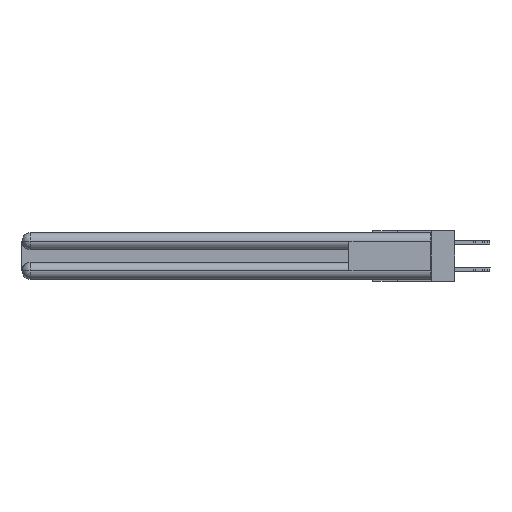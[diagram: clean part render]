
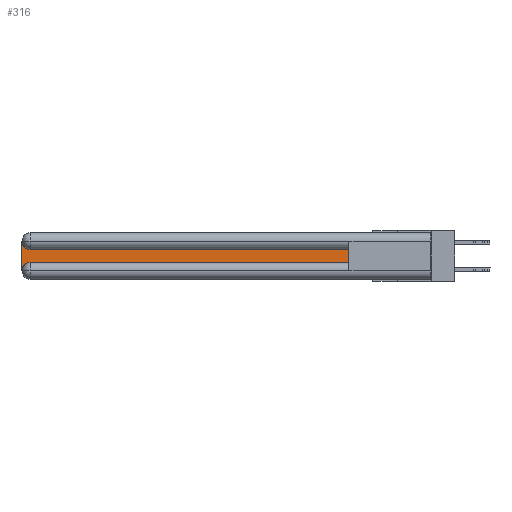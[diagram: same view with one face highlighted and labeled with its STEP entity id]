
A CAD part, left-side view. The second image highlights one B-rep face of the part: STEP entity #316.
In plain terms, the highlighted planar face has unit normal (-1, 0, 0).
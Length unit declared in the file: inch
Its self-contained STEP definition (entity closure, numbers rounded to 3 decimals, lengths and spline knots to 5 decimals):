
#155 = VERTEX_POINT ( 'NONE', #11225 ) ;
#316 = ADVANCED_FACE ( 'NONE', ( #6992 ), #21529, .F. ) ;
#781 = AXIS2_PLACEMENT_3D ( 'NONE', #875, #32327, #5936 ) ;
#875 = CARTESIAN_POINT ( 'NONE',  ( 0.075, 3., -0.1225 ) ) ;
#1065 = LINE ( 'NONE', #25532, #20812 ) ;
#3081 = CARTESIAN_POINT ( 'NONE',  ( 0.075, 3., -0.2775 ) ) ;
#3190 = CARTESIAN_POINT ( 'NONE',  ( 0.075, 2.94, -0.1225 ) ) ;
#3646 = CIRCLE ( 'NONE', #11608, 0.06 ) ;
#3935 = CARTESIAN_POINT ( 'NONE',  ( 0.075, 0.6, -0.1225 ) ) ;
#4728 = DIRECTION ( 'NONE',  ( 0., -1., 0. ) ) ;
#5057 = VERTEX_POINT ( 'NONE', #25517 ) ;
#5254 = ORIENTED_EDGE ( 'NONE', *, *, #30267, .T. ) ;
#5693 = EDGE_CURVE ( 'NONE', #22349, #15448, #27275, .T. ) ;
#5936 = DIRECTION ( 'NONE',  ( 0., 0., -1. ) ) ;
#6857 = ORIENTED_EDGE ( 'NONE', *, *, #26820, .T. ) ;
#6992 = FACE_OUTER_BOUND ( 'NONE', #21489, .T. ) ;
#7317 = CARTESIAN_POINT ( 'NONE',  ( 0.075, 3., -0.0625 ) ) ;
#7376 = CARTESIAN_POINT ( 'NONE',  ( 0.075, 2.94, -0.2775 ) ) ;
#8528 = EDGE_CURVE ( 'NONE', #155, #13102, #28706, .T. ) ;
#10311 = DIRECTION ( 'NONE',  ( 0., 0., -1. ) ) ;
#10368 = DIRECTION ( 'NONE',  ( 1., 0., 0. ) ) ;
#11192 = LINE ( 'NONE', #20145, #24390 ) ;
#11225 = CARTESIAN_POINT ( 'NONE',  ( 0.075, 0.6, -0.2175 ) ) ;
#11458 = ORIENTED_EDGE ( 'NONE', *, *, #5693, .T. ) ;
#11608 = AXIS2_PLACEMENT_3D ( 'NONE', #7376, #30932, #10311 ) ;
#11888 = LINE ( 'NONE', #3935, #13582 ) ;
#13102 = VERTEX_POINT ( 'NONE', #32010 ) ;
#13129 = VERTEX_POINT ( 'NONE', #3081 ) ;
#13582 = VECTOR ( 'NONE', #15214, 39.37008 ) ;
#13713 = AXIS2_PLACEMENT_3D ( 'NONE', #15583, #10368, #28789 ) ;
#15214 = DIRECTION ( 'NONE',  ( 0., 1., 0. ) ) ;
#15448 = VERTEX_POINT ( 'NONE', #7317 ) ;
#15583 = CARTESIAN_POINT ( 'NONE',  ( 0.075, 2.94, -0.0625 ) ) ;
#20145 = CARTESIAN_POINT ( 'NONE',  ( 0.075, 0.6, -0.2175 ) ) ;
#20575 = EDGE_CURVE ( 'NONE', #15448, #13129, #1065, .T. ) ;
#20812 = VECTOR ( 'NONE', #28038, 39.37008 ) ;
#21489 = EDGE_LOOP ( 'NONE', ( #29702, #11458, #33366, #6857, #5254, #27272 ) ) ;
#21529 = PLANE ( 'NONE',  #781 ) ;
#22349 = VERTEX_POINT ( 'NONE', #3190 ) ;
#24390 = VECTOR ( 'NONE', #4728, 39.37008 ) ;
#25517 = CARTESIAN_POINT ( 'NONE',  ( 0.075, 2.94, -0.2175 ) ) ;
#25532 = CARTESIAN_POINT ( 'NONE',  ( 0.075, 3., -0.2175 ) ) ;
#26820 = EDGE_CURVE ( 'NONE', #13129, #5057, #3646, .T. ) ;
#27059 = VECTOR ( 'NONE', #32416, 39.37008 ) ;
#27272 = ORIENTED_EDGE ( 'NONE', *, *, #8528, .T. ) ;
#27275 = CIRCLE ( 'NONE', #13713, 0.06 ) ;
#28038 = DIRECTION ( 'NONE',  ( 0., 0., -1. ) ) ;
#28706 = LINE ( 'NONE', #29772, #27059 ) ;
#28789 = DIRECTION ( 'NONE',  ( 0., 0., -1. ) ) ;
#29702 = ORIENTED_EDGE ( 'NONE', *, *, #31584, .T. ) ;
#29772 = CARTESIAN_POINT ( 'NONE',  ( 0.075, 0.6, -0.2175 ) ) ;
#30267 = EDGE_CURVE ( 'NONE', #5057, #155, #11192, .T. ) ;
#30932 = DIRECTION ( 'NONE',  ( 1., 0., 0. ) ) ;
#31584 = EDGE_CURVE ( 'NONE', #13102, #22349, #11888, .T. ) ;
#32010 = CARTESIAN_POINT ( 'NONE',  ( 0.075, 0.6, -0.1225 ) ) ;
#32327 = DIRECTION ( 'NONE',  ( 1., 0., 0. ) ) ;
#32416 = DIRECTION ( 'NONE',  ( 0., 0., 1. ) ) ;
#33366 = ORIENTED_EDGE ( 'NONE', *, *, #20575, .T. ) ;
